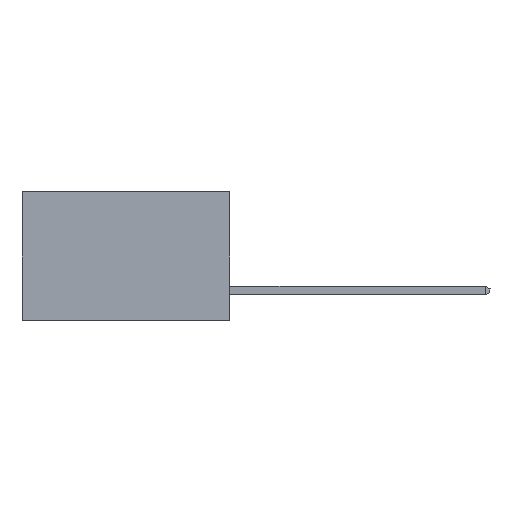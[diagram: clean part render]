
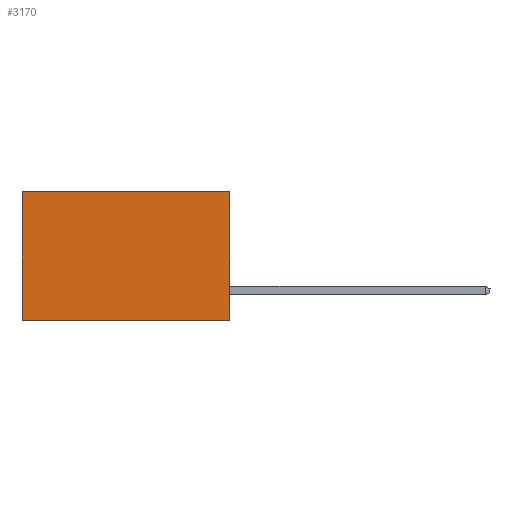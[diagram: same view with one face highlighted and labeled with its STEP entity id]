
A CAD part, left-side view. The second image highlights one B-rep face of the part: STEP entity #3170.
In plain terms, the highlighted planar face has unit normal (-1, 0, 0).
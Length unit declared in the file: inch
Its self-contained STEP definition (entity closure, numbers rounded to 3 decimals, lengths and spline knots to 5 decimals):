
#83 = CARTESIAN_POINT ( 'NONE',  ( 0.2615, 0., -0.37 ) ) ;
#344 = CARTESIAN_POINT ( 'NONE',  ( 0.2615, 0.6, 0. ) ) ;
#697 = VECTOR ( 'NONE', #10486, 39.37008 ) ;
#1191 = DIRECTION ( 'NONE',  ( 0., 0., -1. ) ) ;
#1422 = CARTESIAN_POINT ( 'NONE',  ( 0.2615, 0., -0.37 ) ) ;
#1934 = VERTEX_POINT ( 'NONE', #4588 ) ;
#2503 = LINE ( 'NONE', #3847, #11167 ) ;
#2882 = LINE ( 'NONE', #1422, #697 ) ;
#3170 = ADVANCED_FACE ( 'NONE', ( #9327 ), #4954, .F. ) ;
#3770 = DIRECTION ( 'NONE',  ( 0., 0., -1. ) ) ;
#3792 = VERTEX_POINT ( 'NONE', #344 ) ;
#3836 = DIRECTION ( 'NONE',  ( 1., 0., 0. ) ) ;
#3847 = CARTESIAN_POINT ( 'NONE',  ( 0.2615, 0.6, -0.37 ) ) ;
#3861 = EDGE_CURVE ( 'NONE', #3792, #1934, #2503, .T. ) ;
#3905 = ORIENTED_EDGE ( 'NONE', *, *, #13806, .F. ) ;
#4345 = VECTOR ( 'NONE', #1191, 39.37008 ) ;
#4588 = CARTESIAN_POINT ( 'NONE',  ( 0.2615, 0.6, -0.37 ) ) ;
#4722 = VERTEX_POINT ( 'NONE', #13057 ) ;
#4746 = EDGE_CURVE ( 'NONE', #4722, #3792, #10851, .T. ) ;
#4954 = PLANE ( 'NONE',  #13230 ) ;
#5586 = LINE ( 'NONE', #83, #4345 ) ;
#6278 = VECTOR ( 'NONE', #10552, 39.37008 ) ;
#7912 = ORIENTED_EDGE ( 'NONE', *, *, #3861, .T. ) ;
#8214 = VERTEX_POINT ( 'NONE', #11848 ) ;
#8727 = ORIENTED_EDGE ( 'NONE', *, *, #4746, .T. ) ;
#9327 = FACE_OUTER_BOUND ( 'NONE', #10606, .T. ) ;
#9482 = CARTESIAN_POINT ( 'NONE',  ( 0.2615, 0., -0.37 ) ) ;
#9765 = ORIENTED_EDGE ( 'NONE', *, *, #11595, .F. ) ;
#10486 = DIRECTION ( 'NONE',  ( 0., 1., 0. ) ) ;
#10552 = DIRECTION ( 'NONE',  ( 0., 1., 0. ) ) ;
#10606 = EDGE_LOOP ( 'NONE', ( #7912, #9765, #3905, #8727 ) ) ;
#10851 = LINE ( 'NONE', #14228, #6278 ) ;
#11167 = VECTOR ( 'NONE', #3770, 39.37008 ) ;
#11595 = EDGE_CURVE ( 'NONE', #8214, #1934, #2882, .T. ) ;
#11848 = CARTESIAN_POINT ( 'NONE',  ( 0.2615, 0., -0.37 ) ) ;
#13057 = CARTESIAN_POINT ( 'NONE',  ( 0.2615, 0., 0. ) ) ;
#13230 = AXIS2_PLACEMENT_3D ( 'NONE', #9482, #3836, #13833 ) ;
#13806 = EDGE_CURVE ( 'NONE', #4722, #8214, #5586, .T. ) ;
#13833 = DIRECTION ( 'NONE',  ( 0., 0., -1. ) ) ;
#14228 = CARTESIAN_POINT ( 'NONE',  ( 0.2615, 0., 0. ) ) ;
